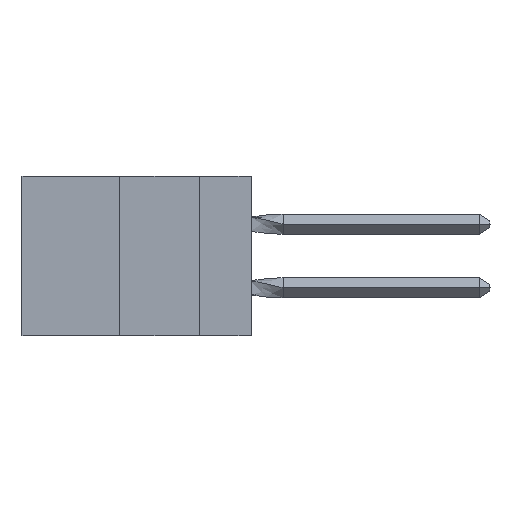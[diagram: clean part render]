
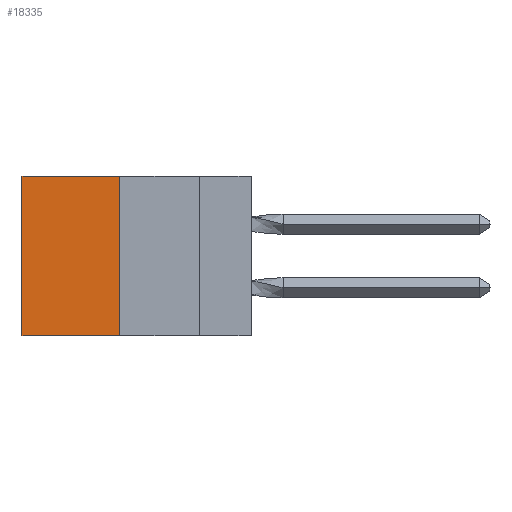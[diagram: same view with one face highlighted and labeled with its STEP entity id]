
A CAD part, left-side view. The second image highlights one B-rep face of the part: STEP entity #18335.
In plain terms, the highlighted planar face has unit normal (-1, 0, 0).
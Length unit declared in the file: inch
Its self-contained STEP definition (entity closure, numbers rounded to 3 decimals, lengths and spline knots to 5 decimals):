
#780 = AXIS2_PLACEMENT_3D ( 'NONE', #26738, #22314, #1726 ) ;
#941 = DIRECTION ( 'NONE',  ( 0., 1., 0. ) ) ;
#961 = VERTEX_POINT ( 'NONE', #21231 ) ;
#1726 = DIRECTION ( 'NONE',  ( 0., 0., -1. ) ) ;
#1732 = CARTESIAN_POINT ( 'NONE',  ( 0.305, 0.413, 0. ) ) ;
#4073 = FACE_OUTER_BOUND ( 'NONE', #5460, .T. ) ;
#4256 = VERTEX_POINT ( 'NONE', #4542 ) ;
#4490 = VERTEX_POINT ( 'NONE', #5035 ) ;
#4542 = CARTESIAN_POINT ( 'NONE',  ( 0.305, 0.413, 0. ) ) ;
#4917 = CARTESIAN_POINT ( 'NONE',  ( 0.305, 0.413, -0.5 ) ) ;
#5035 = CARTESIAN_POINT ( 'NONE',  ( 0.305, 0.72, -0.5 ) ) ;
#5460 = EDGE_LOOP ( 'NONE', ( #25582, #7616, #12393, #28875 ) ) ;
#5933 = VECTOR ( 'NONE', #14695, 39.37008 ) ;
#7616 = ORIENTED_EDGE ( 'NONE', *, *, #21599, .F. ) ;
#8891 = LINE ( 'NONE', #1732, #28849 ) ;
#9121 = VERTEX_POINT ( 'NONE', #28441 ) ;
#11791 = LINE ( 'NONE', #18744, #20723 ) ;
#12393 = ORIENTED_EDGE ( 'NONE', *, *, #20468, .F. ) ;
#14332 = EDGE_CURVE ( 'NONE', #961, #4490, #19563, .T. ) ;
#14695 = DIRECTION ( 'NONE',  ( 0., 0., -1. ) ) ;
#15438 = LINE ( 'NONE', #4917, #23962 ) ;
#18012 = DIRECTION ( 'NONE',  ( 0., 1., 0. ) ) ;
#18335 = ADVANCED_FACE ( 'NONE', ( #4073 ), #20000, .F. ) ;
#18607 = DIRECTION ( 'NONE',  ( 0., 0., -1. ) ) ;
#18744 = CARTESIAN_POINT ( 'NONE',  ( 0.305, 0.413, -0.5 ) ) ;
#19278 = CARTESIAN_POINT ( 'NONE',  ( 0.305, 0.72, -0.5 ) ) ;
#19563 = LINE ( 'NONE', #19278, #5933 ) ;
#20000 = PLANE ( 'NONE',  #780 ) ;
#20468 = EDGE_CURVE ( 'NONE', #4256, #9121, #15438, .T. ) ;
#20723 = VECTOR ( 'NONE', #941, 39.37008 ) ;
#21231 = CARTESIAN_POINT ( 'NONE',  ( 0.305, 0.72, 0. ) ) ;
#21599 = EDGE_CURVE ( 'NONE', #9121, #4490, #11791, .T. ) ;
#21931 = EDGE_CURVE ( 'NONE', #4256, #961, #8891, .T. ) ;
#22314 = DIRECTION ( 'NONE',  ( 1., 0., 0. ) ) ;
#23962 = VECTOR ( 'NONE', #18607, 39.37008 ) ;
#25582 = ORIENTED_EDGE ( 'NONE', *, *, #14332, .T. ) ;
#26738 = CARTESIAN_POINT ( 'NONE',  ( 0.305, 0.413, -0.5 ) ) ;
#28441 = CARTESIAN_POINT ( 'NONE',  ( 0.305, 0.413, -0.5 ) ) ;
#28849 = VECTOR ( 'NONE', #18012, 39.37008 ) ;
#28875 = ORIENTED_EDGE ( 'NONE', *, *, #21931, .T. ) ;
